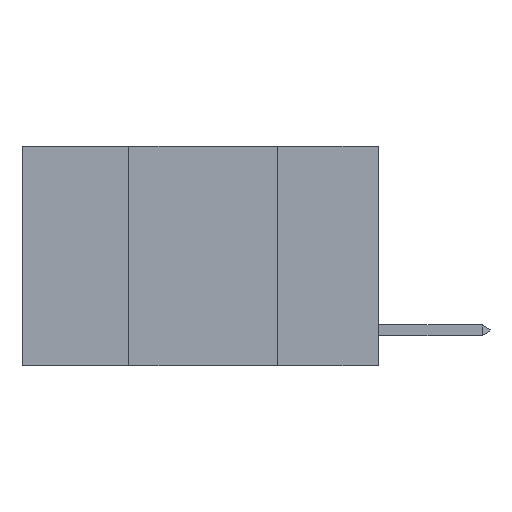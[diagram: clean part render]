
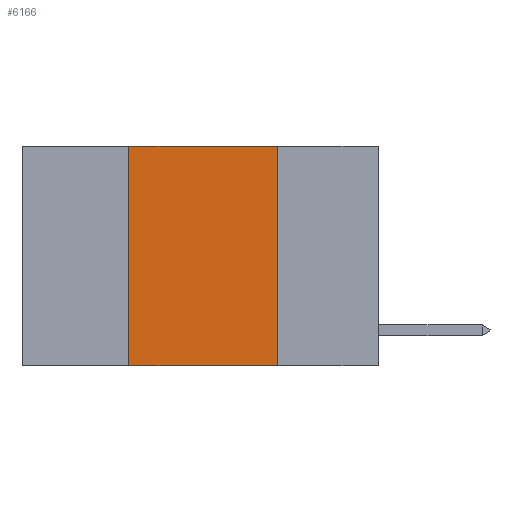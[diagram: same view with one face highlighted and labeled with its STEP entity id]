
A CAD part, left-side view. The second image highlights one B-rep face of the part: STEP entity #6166.
In plain terms, the highlighted planar face has unit normal (-1, 0, 0).
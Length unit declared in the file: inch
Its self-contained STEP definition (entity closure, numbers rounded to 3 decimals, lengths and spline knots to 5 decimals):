
#172 = CARTESIAN_POINT ( 'NONE',  ( 0., 0.6, -0.37 ) ) ;
#1257 = LINE ( 'NONE', #1301, #9758 ) ;
#1301 = CARTESIAN_POINT ( 'NONE',  ( 0., 0.17, 0. ) ) ;
#1561 = ORIENTED_EDGE ( 'NONE', *, *, #8530, .T. ) ;
#2160 = VERTEX_POINT ( 'NONE', #2804 ) ;
#2551 = LINE ( 'NONE', #5273, #8882 ) ;
#2559 = CARTESIAN_POINT ( 'NONE',  ( 0., 0.17, 0. ) ) ;
#2759 = DIRECTION ( 'NONE',  ( 0., 0., 1. ) ) ;
#2804 = CARTESIAN_POINT ( 'NONE',  ( 0., 0.17, -0.37 ) ) ;
#3353 = DIRECTION ( 'NONE',  ( 0., -1., 0. ) ) ;
#3492 = DIRECTION ( 'NONE',  ( 0., 0., -1. ) ) ;
#3605 = VERTEX_POINT ( 'NONE', #6411 ) ;
#3817 = VECTOR ( 'NONE', #3353, 39.37008 ) ;
#3854 = DIRECTION ( 'NONE',  ( 0., 0., -1. ) ) ;
#4572 = ORIENTED_EDGE ( 'NONE', *, *, #8519, .F. ) ;
#4846 = CARTESIAN_POINT ( 'NONE',  ( 0., 0.42, -0.37 ) ) ;
#5020 = EDGE_CURVE ( 'NONE', #3605, #6125, #8212, .T. ) ;
#5273 = CARTESIAN_POINT ( 'NONE',  ( 0., 0.42, 0. ) ) ;
#5301 = DIRECTION ( 'NONE',  ( 0., -1., 0. ) ) ;
#6010 = EDGE_LOOP ( 'NONE', ( #10504, #9620, #4572, #1561 ) ) ;
#6125 = VERTEX_POINT ( 'NONE', #2559 ) ;
#6166 = ADVANCED_FACE ( 'NONE', ( #8937 ), #6786, .F. ) ;
#6411 = CARTESIAN_POINT ( 'NONE',  ( 0., 0.42, 0. ) ) ;
#6646 = CARTESIAN_POINT ( 'NONE',  ( 0., 0.6, 0. ) ) ;
#6786 = PLANE ( 'NONE',  #8660 ) ;
#6937 = EDGE_CURVE ( 'NONE', #6125, #2160, #1257, .T. ) ;
#8212 = LINE ( 'NONE', #6646, #3817 ) ;
#8379 = VECTOR ( 'NONE', #5301, 39.37008 ) ;
#8429 = DIRECTION ( 'NONE',  ( 1., 0., 0. ) ) ;
#8519 = EDGE_CURVE ( 'NONE', #9617, #3605, #2551, .T. ) ;
#8530 = EDGE_CURVE ( 'NONE', #9617, #2160, #10471, .T. ) ;
#8660 = AXIS2_PLACEMENT_3D ( 'NONE', #9147, #8429, #3492 ) ;
#8882 = VECTOR ( 'NONE', #2759, 39.37008 ) ;
#8937 = FACE_OUTER_BOUND ( 'NONE', #6010, .T. ) ;
#9147 = CARTESIAN_POINT ( 'NONE',  ( 0., 0.6, 0. ) ) ;
#9617 = VERTEX_POINT ( 'NONE', #4846 ) ;
#9620 = ORIENTED_EDGE ( 'NONE', *, *, #5020, .F. ) ;
#9758 = VECTOR ( 'NONE', #3854, 39.37008 ) ;
#10471 = LINE ( 'NONE', #172, #8379 ) ;
#10504 = ORIENTED_EDGE ( 'NONE', *, *, #6937, .F. ) ;
